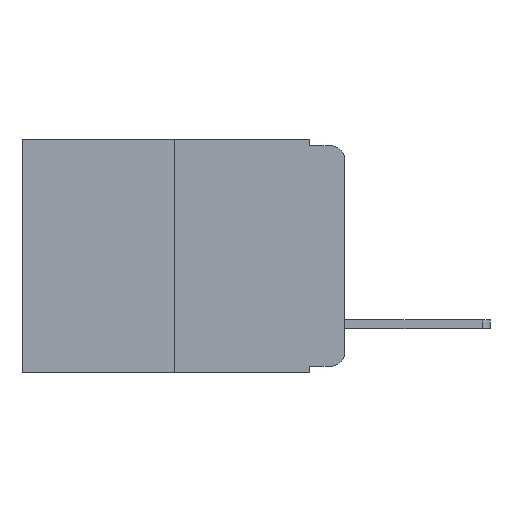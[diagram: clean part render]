
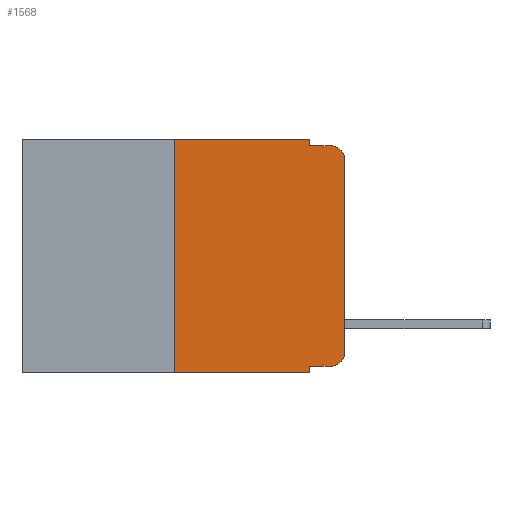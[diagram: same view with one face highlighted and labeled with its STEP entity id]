
A CAD part, left-side view. The second image highlights one B-rep face of the part: STEP entity #1568.
In plain terms, the highlighted planar face has unit normal (-1, 0, 0).
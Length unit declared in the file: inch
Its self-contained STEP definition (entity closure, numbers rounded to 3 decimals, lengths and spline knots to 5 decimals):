
#40 = CIRCLE ( 'NONE', #9431, 0.02 ) ;
#114 = EDGE_CURVE ( 'NONE', #2048, #457, #11068, .T. ) ;
#169 = CARTESIAN_POINT ( 'NONE',  ( 0., 0., -0.03 ) ) ;
#457 = VERTEX_POINT ( 'NONE', #169 ) ;
#458 = CIRCLE ( 'NONE', #4509, 0.02 ) ;
#633 = VECTOR ( 'NONE', #3268, 39.37008 ) ;
#684 = EDGE_CURVE ( 'NONE', #4570, #2355, #7135, .T. ) ;
#711 = ORIENTED_EDGE ( 'NONE', *, *, #1420, .F. ) ;
#748 = VECTOR ( 'NONE', #10366, 39.37008 ) ;
#793 = ORIENTED_EDGE ( 'NONE', *, *, #3354, .T. ) ;
#831 = CARTESIAN_POINT ( 'NONE',  ( 0., 0.051, -0.333 ) ) ;
#1060 = CARTESIAN_POINT ( 'NONE',  ( 0., 0.051, -0.333 ) ) ;
#1109 = ORIENTED_EDGE ( 'NONE', *, *, #11267, .T. ) ;
#1215 = LINE ( 'NONE', #2263, #9954 ) ;
#1420 = EDGE_CURVE ( 'NONE', #10892, #4570, #1215, .T. ) ;
#1443 = ORIENTED_EDGE ( 'NONE', *, *, #2054, .F. ) ;
#1568 = ADVANCED_FACE ( 'NONE', ( #8037 ), #1669, .F. ) ;
#1669 = PLANE ( 'NONE',  #3226 ) ;
#1972 = ORIENTED_EDGE ( 'NONE', *, *, #2714, .F. ) ;
#2048 = VERTEX_POINT ( 'NONE', #7984 ) ;
#2054 = EDGE_CURVE ( 'NONE', #4452, #9336, #9807, .T. ) ;
#2073 = DIRECTION ( 'NONE',  ( 0., 0., -1. ) ) ;
#2177 = VERTEX_POINT ( 'NONE', #5055 ) ;
#2263 = CARTESIAN_POINT ( 'NONE',  ( 0., 0.051, 0. ) ) ;
#2295 = VECTOR ( 'NONE', #3046, 39.37008 ) ;
#2355 = VERTEX_POINT ( 'NONE', #3100 ) ;
#2356 = ORIENTED_EDGE ( 'NONE', *, *, #8793, .F. ) ;
#2415 = DIRECTION ( 'NONE',  ( 0., 0., 1. ) ) ;
#2641 = ORIENTED_EDGE ( 'NONE', *, *, #4002, .T. ) ;
#2683 = CARTESIAN_POINT ( 'NONE',  ( 0., 0.051, 0. ) ) ;
#2714 = EDGE_CURVE ( 'NONE', #5132, #2177, #5068, .T. ) ;
#2770 = DIRECTION ( 'NONE',  ( 0., -1., 0. ) ) ;
#2859 = CARTESIAN_POINT ( 'NONE',  ( 0., 0.051, -0.01 ) ) ;
#3046 = DIRECTION ( 'NONE',  ( 0., 0., 1. ) ) ;
#3100 = CARTESIAN_POINT ( 'NONE',  ( 0., 0.02, -0.01 ) ) ;
#3189 = DIRECTION ( 'NONE',  ( -1., 0., 0. ) ) ;
#3226 = AXIS2_PLACEMENT_3D ( 'NONE', #6085, #10306, #10994 ) ;
#3268 = DIRECTION ( 'NONE',  ( 0., 0., -1. ) ) ;
#3354 = EDGE_CURVE ( 'NONE', #5132, #4748, #10338, .T. ) ;
#3674 = DIRECTION ( 'NONE',  ( 0., -1., 0. ) ) ;
#4002 = EDGE_CURVE ( 'NONE', #4748, #2048, #458, .T. ) ;
#4195 = CARTESIAN_POINT ( 'NONE',  ( 0., 0.02, -0.333 ) ) ;
#4322 = ORIENTED_EDGE ( 'NONE', *, *, #684, .F. ) ;
#4452 = VERTEX_POINT ( 'NONE', #6748 ) ;
#4509 = AXIS2_PLACEMENT_3D ( 'NONE', #4909, #4956, #4946 ) ;
#4570 = VERTEX_POINT ( 'NONE', #8048 ) ;
#4729 = ORIENTED_EDGE ( 'NONE', *, *, #9816, .T. ) ;
#4748 = VERTEX_POINT ( 'NONE', #4195 ) ;
#4829 = ORIENTED_EDGE ( 'NONE', *, *, #114, .T. ) ;
#4909 = CARTESIAN_POINT ( 'NONE',  ( 0., 0.02, -0.313 ) ) ;
#4946 = DIRECTION ( 'NONE',  ( 0., 0., -1. ) ) ;
#4956 = DIRECTION ( 'NONE',  ( -1., 0., 0. ) ) ;
#4962 = CARTESIAN_POINT ( 'NONE',  ( 0., 0.051, 0. ) ) ;
#5055 = CARTESIAN_POINT ( 'NONE',  ( 0., 0.051, -0.343 ) ) ;
#5068 = LINE ( 'NONE', #2683, #633 ) ;
#5132 = VERTEX_POINT ( 'NONE', #831 ) ;
#5353 = VECTOR ( 'NONE', #7217, 39.37008 ) ;
#5512 = EDGE_LOOP ( 'NONE', ( #4829, #4729, #4322, #711, #2356, #1443, #1109, #1972, #793, #2641 ) ) ;
#6072 = CARTESIAN_POINT ( 'NONE',  ( 0., 0.25, 0. ) ) ;
#6085 = CARTESIAN_POINT ( 'NONE',  ( 0., 0.473, 0. ) ) ;
#6380 = CARTESIAN_POINT ( 'NONE',  ( 0., 0.473, 0. ) ) ;
#6748 = CARTESIAN_POINT ( 'NONE',  ( 0., 0.25, -0.343 ) ) ;
#7135 = LINE ( 'NONE', #2859, #9303 ) ;
#7217 = DIRECTION ( 'NONE',  ( 0., -1., 0. ) ) ;
#7901 = VECTOR ( 'NONE', #2415, 39.37008 ) ;
#7923 = LINE ( 'NONE', #8740, #748 ) ;
#7984 = CARTESIAN_POINT ( 'NONE',  ( 0., 0., -0.313 ) ) ;
#8037 = FACE_OUTER_BOUND ( 'NONE', #5512, .T. ) ;
#8048 = CARTESIAN_POINT ( 'NONE',  ( 0., 0.051, -0.01 ) ) ;
#8181 = VECTOR ( 'NONE', #3674, 39.37008 ) ;
#8349 = CARTESIAN_POINT ( 'NONE',  ( 0., 0.02, -0.03 ) ) ;
#8740 = CARTESIAN_POINT ( 'NONE',  ( 0., 0.473, -0.343 ) ) ;
#8793 = EDGE_CURVE ( 'NONE', #9336, #10892, #10013, .T. ) ;
#9030 = CARTESIAN_POINT ( 'NONE',  ( 0., 0., 0. ) ) ;
#9156 = DIRECTION ( 'NONE',  ( 0., 0., -1. ) ) ;
#9303 = VECTOR ( 'NONE', #2770, 39.37008 ) ;
#9336 = VERTEX_POINT ( 'NONE', #6072 ) ;
#9431 = AXIS2_PLACEMENT_3D ( 'NONE', #8349, #3189, #9156 ) ;
#9807 = LINE ( 'NONE', #9974, #7901 ) ;
#9816 = EDGE_CURVE ( 'NONE', #457, #2355, #40, .T. ) ;
#9954 = VECTOR ( 'NONE', #2073, 39.37008 ) ;
#9974 = CARTESIAN_POINT ( 'NONE',  ( 0., 0.25, 0. ) ) ;
#10013 = LINE ( 'NONE', #6380, #5353 ) ;
#10306 = DIRECTION ( 'NONE',  ( 1., 0., 0. ) ) ;
#10338 = LINE ( 'NONE', #1060, #8181 ) ;
#10366 = DIRECTION ( 'NONE',  ( 0., -1., 0. ) ) ;
#10892 = VERTEX_POINT ( 'NONE', #4962 ) ;
#10994 = DIRECTION ( 'NONE',  ( 0., 0., -1. ) ) ;
#11068 = LINE ( 'NONE', #9030, #2295 ) ;
#11267 = EDGE_CURVE ( 'NONE', #4452, #2177, #7923, .T. ) ;
